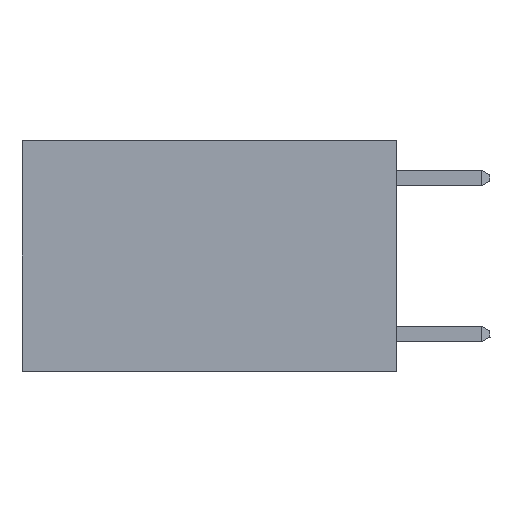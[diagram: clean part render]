
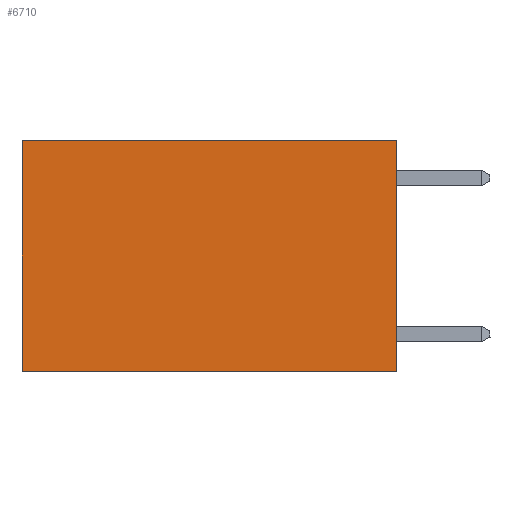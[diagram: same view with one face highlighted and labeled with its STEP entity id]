
A CAD part, left-side view. The second image highlights one B-rep face of the part: STEP entity #6710.
In plain terms, the highlighted planar face has unit normal (-1, 0, 0).
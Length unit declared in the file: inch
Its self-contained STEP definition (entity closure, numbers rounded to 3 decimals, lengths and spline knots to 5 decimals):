
#617 = CARTESIAN_POINT ( 'NONE',  ( 0.2625, 0.6, -0.37 ) ) ;
#1406 = EDGE_LOOP ( 'NONE', ( #8081, #8132, #8329, #8522 ) ) ;
#2808 = LINE ( 'NONE', #20241, #16221 ) ;
#3053 = VERTEX_POINT ( 'NONE', #12648 ) ;
#3511 = VECTOR ( 'NONE', #17510, 39.37008 ) ;
#3632 = LINE ( 'NONE', #15922, #3511 ) ;
#5579 = EDGE_CURVE ( 'NONE', #3053, #6610, #15383, .T. ) ;
#6048 = DIRECTION ( 'NONE',  ( 0., 1., 0. ) ) ;
#6139 = CARTESIAN_POINT ( 'NONE',  ( 0.2625, 0., 0. ) ) ;
#6610 = VERTEX_POINT ( 'NONE', #10576 ) ;
#6710 = ADVANCED_FACE ( 'NONE', ( #6747 ), #8842, .F. ) ;
#6747 = FACE_OUTER_BOUND ( 'NONE', #1406, .T. ) ;
#7011 = DIRECTION ( 'NONE',  ( 0., 1., 0. ) ) ;
#7258 = VERTEX_POINT ( 'NONE', #10216 ) ;
#7511 = AXIS2_PLACEMENT_3D ( 'NONE', #8648, #8644, #8599 ) ;
#8081 = ORIENTED_EDGE ( 'NONE', *, *, #20605, .T. ) ;
#8132 = ORIENTED_EDGE ( 'NONE', *, *, #12437, .F. ) ;
#8329 = ORIENTED_EDGE ( 'NONE', *, *, #16779, .F. ) ;
#8522 = ORIENTED_EDGE ( 'NONE', *, *, #5579, .T. ) ;
#8599 = DIRECTION ( 'NONE',  ( 0., 0., -1. ) ) ;
#8644 = DIRECTION ( 'NONE',  ( 1., 0., 0. ) ) ;
#8648 = CARTESIAN_POINT ( 'NONE',  ( 0.2625, 0., 0. ) ) ;
#8842 = PLANE ( 'NONE',  #7511 ) ;
#10216 = CARTESIAN_POINT ( 'NONE',  ( 0.2625, 0., -0.37 ) ) ;
#10551 = VECTOR ( 'NONE', #13763, 39.37008 ) ;
#10576 = CARTESIAN_POINT ( 'NONE',  ( 0.2625, 0.6, 0. ) ) ;
#10676 = LINE ( 'NONE', #12139, #10551 ) ;
#12139 = CARTESIAN_POINT ( 'NONE',  ( 0.2625, 0., 0. ) ) ;
#12437 = EDGE_CURVE ( 'NONE', #7258, #13044, #2808, .T. ) ;
#12648 = CARTESIAN_POINT ( 'NONE',  ( 0.2625, 0., 0. ) ) ;
#13044 = VERTEX_POINT ( 'NONE', #617 ) ;
#13763 = DIRECTION ( 'NONE',  ( 0., 0., -1. ) ) ;
#15383 = LINE ( 'NONE', #6139, #15441 ) ;
#15441 = VECTOR ( 'NONE', #6048, 39.37008 ) ;
#15922 = CARTESIAN_POINT ( 'NONE',  ( 0.2625, 0.6, 0. ) ) ;
#16221 = VECTOR ( 'NONE', #7011, 39.37008 ) ;
#16779 = EDGE_CURVE ( 'NONE', #3053, #7258, #10676, .T. ) ;
#17510 = DIRECTION ( 'NONE',  ( 0., 0., -1. ) ) ;
#20241 = CARTESIAN_POINT ( 'NONE',  ( 0.2625, 0., -0.37 ) ) ;
#20605 = EDGE_CURVE ( 'NONE', #6610, #13044, #3632, .T. ) ;
